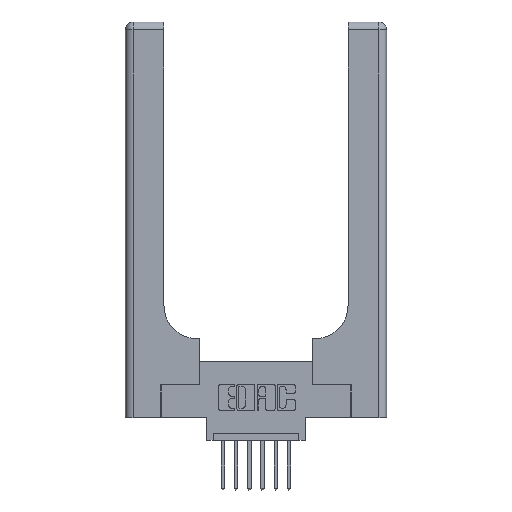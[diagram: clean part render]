
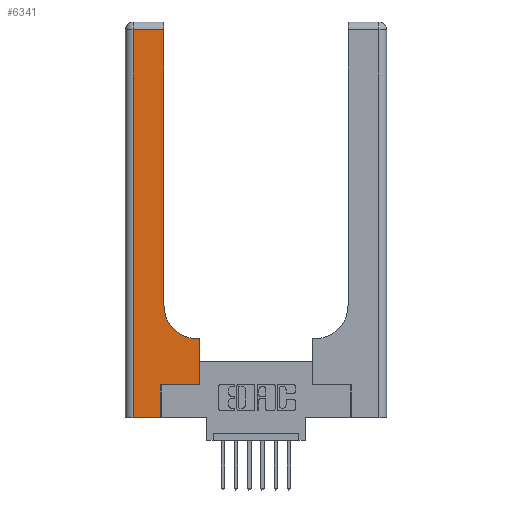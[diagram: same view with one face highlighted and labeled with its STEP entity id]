
A CAD part, top view. The second image highlights one B-rep face of the part: STEP entity #6341.
In plain terms, the highlighted planar face has unit normal (0, 0, 1).
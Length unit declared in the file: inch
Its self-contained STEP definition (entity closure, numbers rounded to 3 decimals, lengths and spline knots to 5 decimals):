
#81 = EDGE_CURVE ( 'NONE', #14103, #10257, #3914, .T. ) ;
#369 = LINE ( 'NONE', #1802, #740 ) ;
#496 = ORIENTED_EDGE ( 'NONE', *, *, #7509, .T. ) ;
#740 = VECTOR ( 'NONE', #6373, 39.37008 ) ;
#972 = LINE ( 'NONE', #11594, #4630 ) ;
#1184 = VECTOR ( 'NONE', #1189, 39.37008 ) ;
#1189 = DIRECTION ( 'NONE',  ( -1., 0., 0. ) ) ;
#1502 = CARTESIAN_POINT ( 'NONE',  ( 0.2915, 2.94, 0.37 ) ) ;
#1546 = LINE ( 'NONE', #7552, #3880 ) ;
#1765 = ORIENTED_EDGE ( 'NONE', *, *, #6872, .T. ) ;
#1802 = CARTESIAN_POINT ( 'NONE',  ( 0.2915, 0.6, 0.37 ) ) ;
#1803 = CARTESIAN_POINT ( 'NONE',  ( 0.5415, 0.6, 0.37 ) ) ;
#1812 = CARTESIAN_POINT ( 'NONE',  ( 0.269, 0.25, 0.37 ) ) ;
#1817 = VERTEX_POINT ( 'NONE', #13917 ) ;
#2013 = EDGE_CURVE ( 'NONE', #14348, #11055, #3446, .T. ) ;
#2191 = ORIENTED_EDGE ( 'NONE', *, *, #4259, .T. ) ;
#2224 = ORIENTED_EDGE ( 'NONE', *, *, #10049, .T. ) ;
#2618 = ORIENTED_EDGE ( 'NONE', *, *, #11197, .T. ) ;
#2678 = DIRECTION ( 'NONE',  ( 0., 0., -1. ) ) ;
#2948 = VECTOR ( 'NONE', #6151, 39.37008 ) ;
#3066 = DIRECTION ( 'NONE',  ( 0., 1., 0. ) ) ;
#3402 = DIRECTION ( 'NONE',  ( 1., 0., 0. ) ) ;
#3446 = LINE ( 'NONE', #1812, #9837 ) ;
#3682 = DIRECTION ( 'NONE',  ( 1., 0., 0. ) ) ;
#3843 = CARTESIAN_POINT ( 'NONE',  ( 0., 0., 0.37 ) ) ;
#3880 = VECTOR ( 'NONE', #13895, 39.37008 ) ;
#3914 = LINE ( 'NONE', #5094, #2948 ) ;
#4091 = CARTESIAN_POINT ( 'NONE',  ( 0.269, 0., 0.37 ) ) ;
#4259 = EDGE_CURVE ( 'NONE', #12857, #14348, #7510, .T. ) ;
#4346 = ORIENTED_EDGE ( 'NONE', *, *, #2013, .T. ) ;
#4495 = VECTOR ( 'NONE', #3066, 39.37008 ) ;
#4630 = VECTOR ( 'NONE', #9889, 39.37008 ) ;
#4783 = EDGE_CURVE ( 'NONE', #1817, #13505, #369, .T. ) ;
#4945 = DIRECTION ( 'NONE',  ( -1., 0., 0. ) ) ;
#5094 = CARTESIAN_POINT ( 'NONE',  ( 0.06, 3., 0.37 ) ) ;
#5155 = CARTESIAN_POINT ( 'NONE',  ( 0.06, 0., 0.37 ) ) ;
#5997 = ORIENTED_EDGE ( 'NONE', *, *, #4783, .T. ) ;
#6151 = DIRECTION ( 'NONE',  ( 0., -1., 0. ) ) ;
#6341 = ADVANCED_FACE ( 'NONE', ( #9230 ), #12842, .F. ) ;
#6373 = DIRECTION ( 'NONE',  ( -1., 0., 0. ) ) ;
#6872 = EDGE_CURVE ( 'NONE', #12770, #12601, #1546, .T. ) ;
#6933 = CIRCLE ( 'NONE', #9325, 0.25 ) ;
#7509 = EDGE_CURVE ( 'NONE', #10257, #12857, #8506, .T. ) ;
#7510 = LINE ( 'NONE', #4091, #4495 ) ;
#7552 = CARTESIAN_POINT ( 'NONE',  ( 0.2915, 3., 0.37 ) ) ;
#8086 = DIRECTION ( 'NONE',  ( 0., 0., -1. ) ) ;
#8506 = LINE ( 'NONE', #3843, #9588 ) ;
#9161 = EDGE_CURVE ( 'NONE', #11055, #1817, #972, .T. ) ;
#9230 = FACE_OUTER_BOUND ( 'NONE', #12082, .T. ) ;
#9325 = AXIS2_PLACEMENT_3D ( 'NONE', #10204, #8086, #3402 ) ;
#9588 = VECTOR ( 'NONE', #3682, 39.37008 ) ;
#9661 = ORIENTED_EDGE ( 'NONE', *, *, #81, .T. ) ;
#9819 = CARTESIAN_POINT ( 'NONE',  ( 0.2915, 0.85, 0.37 ) ) ;
#9837 = VECTOR ( 'NONE', #10903, 39.37008 ) ;
#9889 = DIRECTION ( 'NONE',  ( 0., 1., 0. ) ) ;
#10049 = EDGE_CURVE ( 'NONE', #13505, #12770, #6933, .T. ) ;
#10055 = AXIS2_PLACEMENT_3D ( 'NONE', #13897, #2678, #4945 ) ;
#10204 = CARTESIAN_POINT ( 'NONE',  ( 0.5415, 0.85, 0.37 ) ) ;
#10257 = VERTEX_POINT ( 'NONE', #5155 ) ;
#10903 = DIRECTION ( 'NONE',  ( 1., 0., 0. ) ) ;
#11055 = VERTEX_POINT ( 'NONE', #14593 ) ;
#11197 = EDGE_CURVE ( 'NONE', #12601, #14103, #14678, .T. ) ;
#11594 = CARTESIAN_POINT ( 'NONE',  ( 0.5585, 0.25, 0.37 ) ) ;
#12047 = CARTESIAN_POINT ( 'NONE',  ( 0.269, 0., 0.37 ) ) ;
#12082 = EDGE_LOOP ( 'NONE', ( #1765, #2618, #9661, #496, #2191, #4346, #13706, #5997, #2224 ) ) ;
#12601 = VERTEX_POINT ( 'NONE', #1502 ) ;
#12770 = VERTEX_POINT ( 'NONE', #9819 ) ;
#12813 = CARTESIAN_POINT ( 'NONE',  ( 0.269, 0.25, 0.37 ) ) ;
#12842 = PLANE ( 'NONE',  #10055 ) ;
#12857 = VERTEX_POINT ( 'NONE', #12047 ) ;
#12882 = CARTESIAN_POINT ( 'NONE',  ( 0.06, 2.94, 0.37 ) ) ;
#13505 = VERTEX_POINT ( 'NONE', #1803 ) ;
#13706 = ORIENTED_EDGE ( 'NONE', *, *, #9161, .T. ) ;
#13782 = CARTESIAN_POINT ( 'NONE',  ( 0., 2.94, 0.37 ) ) ;
#13895 = DIRECTION ( 'NONE',  ( 0., 1., 0. ) ) ;
#13897 = CARTESIAN_POINT ( 'NONE',  ( 0., 3., 0.37 ) ) ;
#13917 = CARTESIAN_POINT ( 'NONE',  ( 0.5585, 0.6, 0.37 ) ) ;
#14103 = VERTEX_POINT ( 'NONE', #12882 ) ;
#14348 = VERTEX_POINT ( 'NONE', #12813 ) ;
#14593 = CARTESIAN_POINT ( 'NONE',  ( 0.5585, 0.25, 0.37 ) ) ;
#14678 = LINE ( 'NONE', #13782, #1184 ) ;
